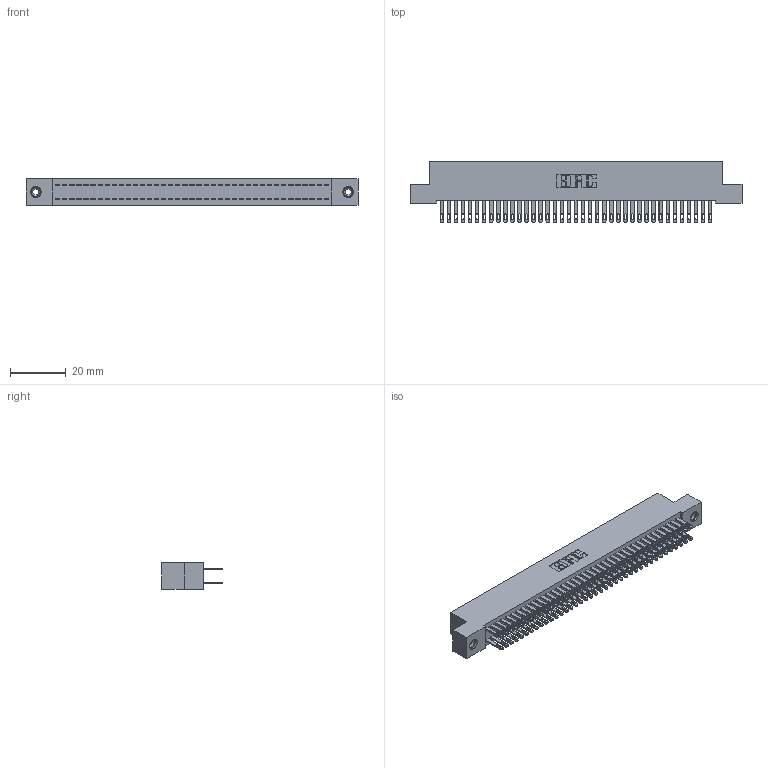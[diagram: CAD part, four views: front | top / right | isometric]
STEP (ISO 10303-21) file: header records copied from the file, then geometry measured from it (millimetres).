
FILE_DESCRIPTION (( 'STEP AP203' ), '1' );
FILE_NAME ('342-078-500-208.STEP', '2018-08-13T13:02:23', ( '' ), ( '' ), 'SwSTEP 2.0', 'SolidWorks 2016', '' );
FILE_SCHEMA (( 'CONFIG_CONTROL_DESIGN' ));
Length unit declared in the file: inch
Products named in the file (4): 345-292-001_345-293-100; 345-250-001_345-250-003-102; 342-078-500-208; 342 Part_TI
Assembly tree (81 placements, depth 2):
  342-078-500-208
    342 Part_TI
    345-292-001_345-293-100  x78
    345-250-001_345-250-003-102  x2
Bounding box: 119.38 x 21.85 x 9.4 mm (x, y, z)
Volume: 10944.7 mm3; surface area: 18498.5 mm2
Topology: 81 solids, 81 shells, 3914 faces, 11901 edges, 7926 vertices
Faces by surface type: plane 2438, cylinder 1460, cone 12, torus 4
Entity records: 26462 total; most frequent: CARTESIAN_POINT 4369, ORIENTED_EDGE 4298, DIRECTION 3771, EDGE_CURVE 2149, LINE 1997, VECTOR 1997, VERTEX_POINT 1428, AXIS2_PLACEMENT_3D 887
